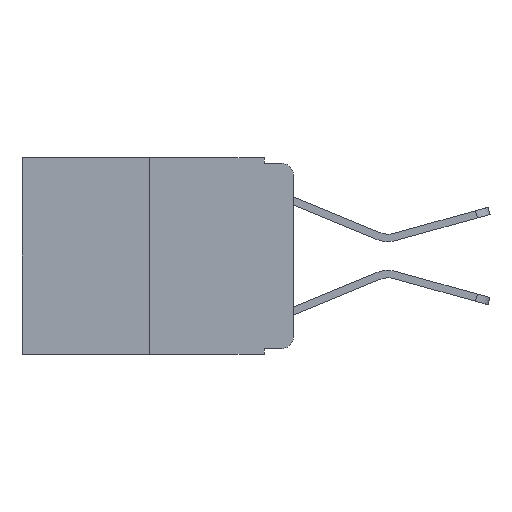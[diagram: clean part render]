
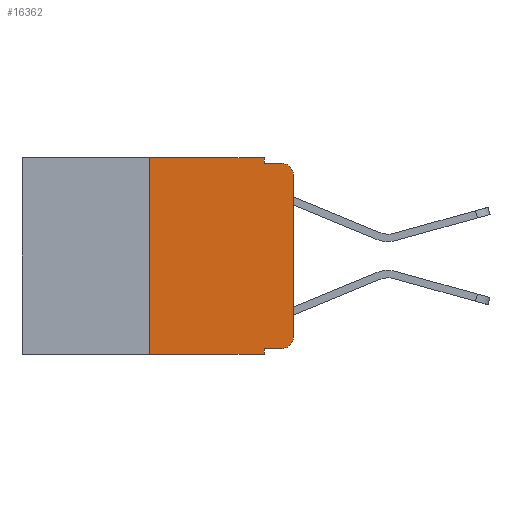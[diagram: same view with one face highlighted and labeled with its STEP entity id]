
A CAD part, left-side view. The second image highlights one B-rep face of the part: STEP entity #16362.
In plain terms, the highlighted planar face has unit normal (-1, 0, 0).
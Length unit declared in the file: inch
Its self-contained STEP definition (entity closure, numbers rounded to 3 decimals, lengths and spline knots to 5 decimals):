
#21 = AXIS2_PLACEMENT_3D ( 'NONE', #8823, #1151, #14145 ) ;
#102 = CARTESIAN_POINT ( 'NONE',  ( 0., 0.051, -0.333 ) ) ;
#336 = CARTESIAN_POINT ( 'NONE',  ( 0., 0.051, -0.343 ) ) ;
#996 = CIRCLE ( 'NONE', #13857, 0.02 ) ;
#1151 = DIRECTION ( 'NONE',  ( 1., 0., 0. ) ) ;
#1950 = CIRCLE ( 'NONE', #22059, 0.02 ) ;
#2252 = EDGE_CURVE ( 'NONE', #4696, #7472, #10655, .T. ) ;
#2581 = EDGE_CURVE ( 'NONE', #6447, #18528, #996, .T. ) ;
#2674 = CARTESIAN_POINT ( 'NONE',  ( 0., 0.051, 0. ) ) ;
#3018 = CARTESIAN_POINT ( 'NONE',  ( 0., 0.02, -0.03 ) ) ;
#3034 = CARTESIAN_POINT ( 'NONE',  ( 0., 0.051, 0. ) ) ;
#3139 = DIRECTION ( 'NONE',  ( -1., 0., 0. ) ) ;
#3606 = VECTOR ( 'NONE', #20353, 39.37008 ) ;
#4696 = VERTEX_POINT ( 'NONE', #16697 ) ;
#5320 = CARTESIAN_POINT ( 'NONE',  ( 0., 0.25, 0. ) ) ;
#5814 = VERTEX_POINT ( 'NONE', #10487 ) ;
#6021 = DIRECTION ( 'NONE',  ( 0., 0., -1. ) ) ;
#6447 = VERTEX_POINT ( 'NONE', #12920 ) ;
#7238 = EDGE_CURVE ( 'NONE', #9711, #20440, #12613, .T. ) ;
#7302 = VECTOR ( 'NONE', #10275, 39.37008 ) ;
#7472 = VERTEX_POINT ( 'NONE', #15627 ) ;
#8289 = CARTESIAN_POINT ( 'NONE',  ( 0., 0.051, 0. ) ) ;
#8312 = ORIENTED_EDGE ( 'NONE', *, *, #22023, .F. ) ;
#8347 = DIRECTION ( 'NONE',  ( 0., -1., 0. ) ) ;
#8767 = VERTEX_POINT ( 'NONE', #5320 ) ;
#8823 = CARTESIAN_POINT ( 'NONE',  ( 0., 0.473, 0. ) ) ;
#8845 = ORIENTED_EDGE ( 'NONE', *, *, #12041, .F. ) ;
#9711 = VERTEX_POINT ( 'NONE', #102 ) ;
#9910 = ORIENTED_EDGE ( 'NONE', *, *, #2252, .F. ) ;
#10063 = VECTOR ( 'NONE', #8347, 39.37008 ) ;
#10275 = DIRECTION ( 'NONE',  ( 0., 0., -1. ) ) ;
#10487 = CARTESIAN_POINT ( 'NONE',  ( 0., 0., -0.03 ) ) ;
#10655 = LINE ( 'NONE', #18376, #15080 ) ;
#10668 = DIRECTION ( 'NONE',  ( 0., 0., -1. ) ) ;
#10806 = VERTEX_POINT ( 'NONE', #15817 ) ;
#10993 = EDGE_CURVE ( 'NONE', #8767, #14719, #14393, .T. ) ;
#11491 = ORIENTED_EDGE ( 'NONE', *, *, #18601, .T. ) ;
#12041 = EDGE_CURVE ( 'NONE', #14719, #4696, #23540, .T. ) ;
#12242 = CARTESIAN_POINT ( 'NONE',  ( 0., 0.25, 0. ) ) ;
#12439 = DIRECTION ( 'NONE',  ( 0., -1., 0. ) ) ;
#12613 = LINE ( 'NONE', #2674, #15222 ) ;
#12920 = CARTESIAN_POINT ( 'NONE',  ( 0., 0.02, -0.333 ) ) ;
#13857 = AXIS2_PLACEMENT_3D ( 'NONE', #17732, #23261, #6021 ) ;
#14145 = DIRECTION ( 'NONE',  ( 0., 0., -1. ) ) ;
#14218 = ORIENTED_EDGE ( 'NONE', *, *, #2581, .T. ) ;
#14319 = EDGE_LOOP ( 'NONE', ( #23314, #20963, #9910, #8845, #21712, #8312, #14485, #18193, #11491, #14218 ) ) ;
#14393 = LINE ( 'NONE', #21956, #10063 ) ;
#14485 = ORIENTED_EDGE ( 'NONE', *, *, #22754, .T. ) ;
#14719 = VERTEX_POINT ( 'NONE', #3034 ) ;
#15010 = CARTESIAN_POINT ( 'NONE',  ( 0., 0.473, -0.343 ) ) ;
#15080 = VECTOR ( 'NONE', #12439, 39.37008 ) ;
#15222 = VECTOR ( 'NONE', #20290, 39.37008 ) ;
#15627 = CARTESIAN_POINT ( 'NONE',  ( 0., 0.02, -0.01 ) ) ;
#15674 = DIRECTION ( 'NONE',  ( 0., 0., 1. ) ) ;
#15817 = CARTESIAN_POINT ( 'NONE',  ( 0., 0.25, -0.343 ) ) ;
#16110 = LINE ( 'NONE', #24020, #3606 ) ;
#16362 = ADVANCED_FACE ( 'NONE', ( #20402 ), #20172, .F. ) ;
#16697 = CARTESIAN_POINT ( 'NONE',  ( 0., 0.051, -0.01 ) ) ;
#16901 = LINE ( 'NONE', #15010, #18435 ) ;
#17732 = CARTESIAN_POINT ( 'NONE',  ( 0., 0.02, -0.313 ) ) ;
#18193 = ORIENTED_EDGE ( 'NONE', *, *, #7238, .F. ) ;
#18194 = EDGE_CURVE ( 'NONE', #5814, #7472, #1950, .T. ) ;
#18376 = CARTESIAN_POINT ( 'NONE',  ( 0., 0.051, -0.01 ) ) ;
#18435 = VECTOR ( 'NONE', #22676, 39.37008 ) ;
#18528 = VERTEX_POINT ( 'NONE', #21144 ) ;
#18601 = EDGE_CURVE ( 'NONE', #9711, #6447, #16110, .T. ) ;
#19352 = VECTOR ( 'NONE', #15674, 39.37008 ) ;
#19660 = VECTOR ( 'NONE', #22660, 39.37008 ) ;
#20172 = PLANE ( 'NONE',  #21 ) ;
#20290 = DIRECTION ( 'NONE',  ( 0., 0., -1. ) ) ;
#20353 = DIRECTION ( 'NONE',  ( 0., -1., 0. ) ) ;
#20402 = FACE_OUTER_BOUND ( 'NONE', #14319, .T. ) ;
#20440 = VERTEX_POINT ( 'NONE', #336 ) ;
#20963 = ORIENTED_EDGE ( 'NONE', *, *, #18194, .T. ) ;
#21144 = CARTESIAN_POINT ( 'NONE',  ( 0., 0., -0.313 ) ) ;
#21712 = ORIENTED_EDGE ( 'NONE', *, *, #10993, .F. ) ;
#21956 = CARTESIAN_POINT ( 'NONE',  ( 0., 0.473, 0. ) ) ;
#22023 = EDGE_CURVE ( 'NONE', #10806, #8767, #23587, .T. ) ;
#22059 = AXIS2_PLACEMENT_3D ( 'NONE', #3018, #3139, #10668 ) ;
#22660 = DIRECTION ( 'NONE',  ( 0., 0., 1. ) ) ;
#22676 = DIRECTION ( 'NONE',  ( 0., -1., 0. ) ) ;
#22754 = EDGE_CURVE ( 'NONE', #10806, #20440, #16901, .T. ) ;
#23036 = LINE ( 'NONE', #23149, #19660 ) ;
#23149 = CARTESIAN_POINT ( 'NONE',  ( 0., 0., 0. ) ) ;
#23261 = DIRECTION ( 'NONE',  ( -1., 0., 0. ) ) ;
#23314 = ORIENTED_EDGE ( 'NONE', *, *, #23899, .T. ) ;
#23540 = LINE ( 'NONE', #8289, #7302 ) ;
#23587 = LINE ( 'NONE', #12242, #19352 ) ;
#23899 = EDGE_CURVE ( 'NONE', #18528, #5814, #23036, .T. ) ;
#24020 = CARTESIAN_POINT ( 'NONE',  ( 0., 0.051, -0.333 ) ) ;
